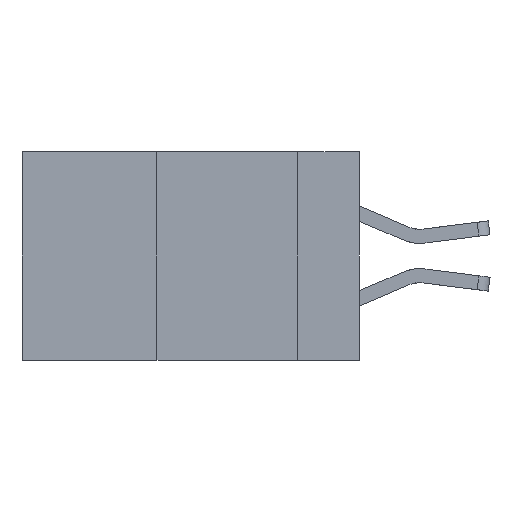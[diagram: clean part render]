
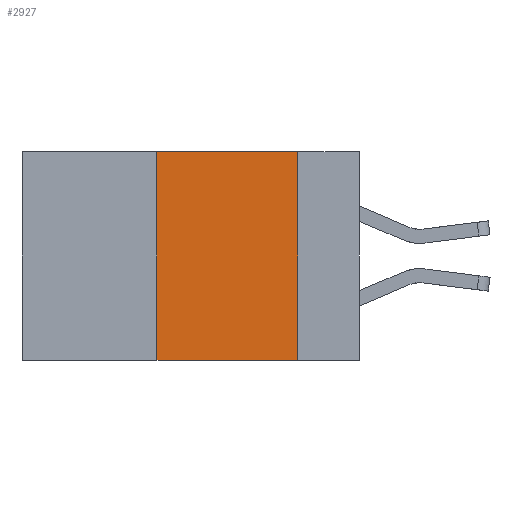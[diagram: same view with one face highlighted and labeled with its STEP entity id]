
A CAD part, left-side view. The second image highlights one B-rep face of the part: STEP entity #2927.
In plain terms, the highlighted planar face has unit normal (-1, 0, 0).
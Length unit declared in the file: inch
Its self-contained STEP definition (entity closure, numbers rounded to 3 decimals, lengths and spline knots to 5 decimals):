
#137 = LINE ( 'NONE', #1113, #8415 ) ;
#482 = CARTESIAN_POINT ( 'NONE',  ( 0., 0.6, -0.37 ) ) ;
#1113 = CARTESIAN_POINT ( 'NONE',  ( 0., 0.6, 0. ) ) ;
#1132 = AXIS2_PLACEMENT_3D ( 'NONE', #9083, #9017, #9011 ) ;
#1186 = CARTESIAN_POINT ( 'NONE',  ( 0., 0.11, 0. ) ) ;
#1346 = DIRECTION ( 'NONE',  ( 0., -1., 0. ) ) ;
#1500 = CARTESIAN_POINT ( 'NONE',  ( 0., 0.36, 0. ) ) ;
#1680 = ORIENTED_EDGE ( 'NONE', *, *, #8156, .F. ) ;
#2753 = EDGE_CURVE ( 'NONE', #8212, #3420, #6666, .T. ) ;
#2927 = ADVANCED_FACE ( 'NONE', ( #9344 ), #9093, .F. ) ;
#3351 = LINE ( 'NONE', #482, #7707 ) ;
#3420 = VERTEX_POINT ( 'NONE', #6643 ) ;
#3653 = ORIENTED_EDGE ( 'NONE', *, *, #2753, .F. ) ;
#3705 = DIRECTION ( 'NONE',  ( 0., 0., 1. ) ) ;
#3723 = CARTESIAN_POINT ( 'NONE',  ( 0., 0.36, 0. ) ) ;
#3900 = EDGE_CURVE ( 'NONE', #6273, #4292, #8859, .T. ) ;
#3918 = ORIENTED_EDGE ( 'NONE', *, *, #3900, .F. ) ;
#4292 = VERTEX_POINT ( 'NONE', #1500 ) ;
#4491 = VECTOR ( 'NONE', #10146, 39.37008 ) ;
#4604 = VECTOR ( 'NONE', #3705, 39.37008 ) ;
#4946 = CARTESIAN_POINT ( 'NONE',  ( 0., 0.36, -0.37 ) ) ;
#5923 = EDGE_LOOP ( 'NONE', ( #3653, #1680, #3918, #8229 ) ) ;
#6124 = EDGE_CURVE ( 'NONE', #6273, #3420, #3351, .T. ) ;
#6273 = VERTEX_POINT ( 'NONE', #4946 ) ;
#6643 = CARTESIAN_POINT ( 'NONE',  ( 0., 0.11, -0.37 ) ) ;
#6666 = LINE ( 'NONE', #10131, #4491 ) ;
#7707 = VECTOR ( 'NONE', #1346, 39.37008 ) ;
#8156 = EDGE_CURVE ( 'NONE', #4292, #8212, #137, .T. ) ;
#8212 = VERTEX_POINT ( 'NONE', #1186 ) ;
#8229 = ORIENTED_EDGE ( 'NONE', *, *, #6124, .T. ) ;
#8415 = VECTOR ( 'NONE', #8522, 39.37008 ) ;
#8522 = DIRECTION ( 'NONE',  ( 0., -1., 0. ) ) ;
#8859 = LINE ( 'NONE', #3723, #4604 ) ;
#9011 = DIRECTION ( 'NONE',  ( 0., 0., -1. ) ) ;
#9017 = DIRECTION ( 'NONE',  ( 1., 0., 0. ) ) ;
#9083 = CARTESIAN_POINT ( 'NONE',  ( 0., 0.6, 0. ) ) ;
#9093 = PLANE ( 'NONE',  #1132 ) ;
#9344 = FACE_OUTER_BOUND ( 'NONE', #5923, .T. ) ;
#10131 = CARTESIAN_POINT ( 'NONE',  ( 0., 0.11, 0. ) ) ;
#10146 = DIRECTION ( 'NONE',  ( 0., 0., -1. ) ) ;
